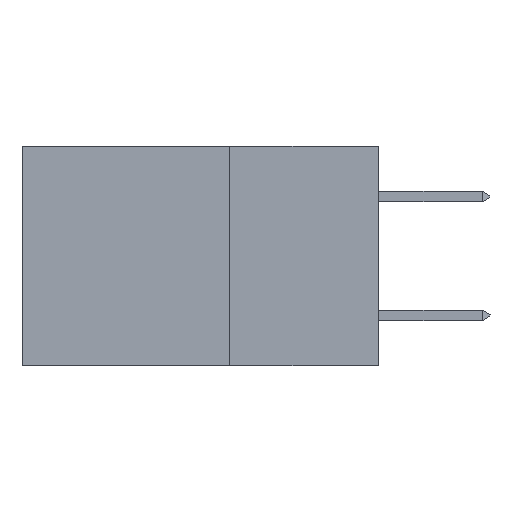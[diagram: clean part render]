
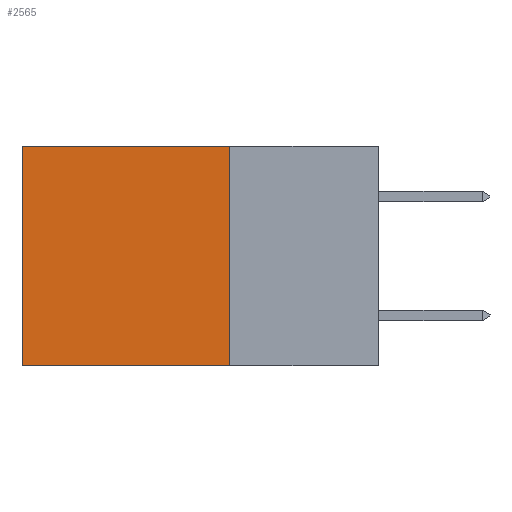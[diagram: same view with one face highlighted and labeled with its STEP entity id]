
A CAD part, left-side view. The second image highlights one B-rep face of the part: STEP entity #2565.
In plain terms, the highlighted planar face has unit normal (-1, 0, 0).
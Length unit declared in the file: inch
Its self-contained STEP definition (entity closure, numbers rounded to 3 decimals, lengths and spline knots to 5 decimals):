
#1062 = CARTESIAN_POINT ( 'NONE',  ( 0.298, 0.6, 0. ) ) ;
#1147 = VERTEX_POINT ( 'NONE', #3319 ) ;
#1217 = CARTESIAN_POINT ( 'NONE',  ( 0.298, 0.25, 0. ) ) ;
#1402 = DIRECTION ( 'NONE',  ( 1., 0., 0. ) ) ;
#2479 = DIRECTION ( 'NONE',  ( 0., 1., 0. ) ) ;
#2565 = ADVANCED_FACE ( 'NONE', ( #6743 ), #9549, .F. ) ;
#2933 = ORIENTED_EDGE ( 'NONE', *, *, #21129, .F. ) ;
#3153 = ORIENTED_EDGE ( 'NONE', *, *, #9541, .F. ) ;
#3319 = CARTESIAN_POINT ( 'NONE',  ( 0.298, 0.6, -0.37 ) ) ;
#4334 = EDGE_LOOP ( 'NONE', ( #25631, #3153, #2933, #25802 ) ) ;
#4540 = LINE ( 'NONE', #23765, #10649 ) ;
#6743 = FACE_OUTER_BOUND ( 'NONE', #4334, .T. ) ;
#7391 = DIRECTION ( 'NONE',  ( 0., 0., -1. ) ) ;
#9336 = CARTESIAN_POINT ( 'NONE',  ( 0.298, 0.25, 0. ) ) ;
#9501 = AXIS2_PLACEMENT_3D ( 'NONE', #1217, #1402, #21641 ) ;
#9541 = EDGE_CURVE ( 'NONE', #10782, #1147, #24014, .T. ) ;
#9549 = PLANE ( 'NONE',  #9501 ) ;
#10601 = VECTOR ( 'NONE', #7391, 39.37008 ) ;
#10649 = VECTOR ( 'NONE', #11219, 39.37008 ) ;
#10782 = VERTEX_POINT ( 'NONE', #19800 ) ;
#11219 = DIRECTION ( 'NONE',  ( 0., 0., -1. ) ) ;
#12501 = VERTEX_POINT ( 'NONE', #12600 ) ;
#12600 = CARTESIAN_POINT ( 'NONE',  ( 0.298, 0.25, 0. ) ) ;
#13626 = EDGE_CURVE ( 'NONE', #20836, #1147, #14788, .T. ) ;
#14788 = LINE ( 'NONE', #1062, #10601 ) ;
#15524 = VECTOR ( 'NONE', #2479, 39.37008 ) ;
#16477 = CARTESIAN_POINT ( 'NONE',  ( 0.298, 0.6, 0. ) ) ;
#18770 = VECTOR ( 'NONE', #23865, 39.37008 ) ;
#19800 = CARTESIAN_POINT ( 'NONE',  ( 0.298, 0.25, -0.37 ) ) ;
#20836 = VERTEX_POINT ( 'NONE', #16477 ) ;
#21129 = EDGE_CURVE ( 'NONE', #12501, #10782, #4540, .T. ) ;
#21641 = DIRECTION ( 'NONE',  ( 0., 0., -1. ) ) ;
#22902 = CARTESIAN_POINT ( 'NONE',  ( 0.298, 0.25, -0.37 ) ) ;
#23005 = LINE ( 'NONE', #9336, #18770 ) ;
#23765 = CARTESIAN_POINT ( 'NONE',  ( 0.298, 0.25, 0. ) ) ;
#23865 = DIRECTION ( 'NONE',  ( 0., 1., 0. ) ) ;
#24014 = LINE ( 'NONE', #22902, #15524 ) ;
#24911 = EDGE_CURVE ( 'NONE', #12501, #20836, #23005, .T. ) ;
#25631 = ORIENTED_EDGE ( 'NONE', *, *, #13626, .T. ) ;
#25802 = ORIENTED_EDGE ( 'NONE', *, *, #24911, .T. ) ;
